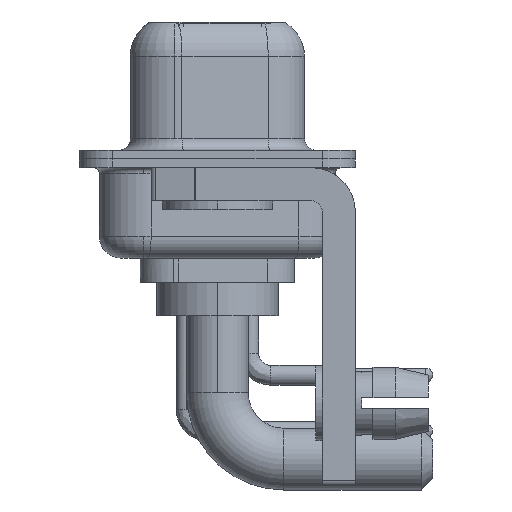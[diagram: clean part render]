
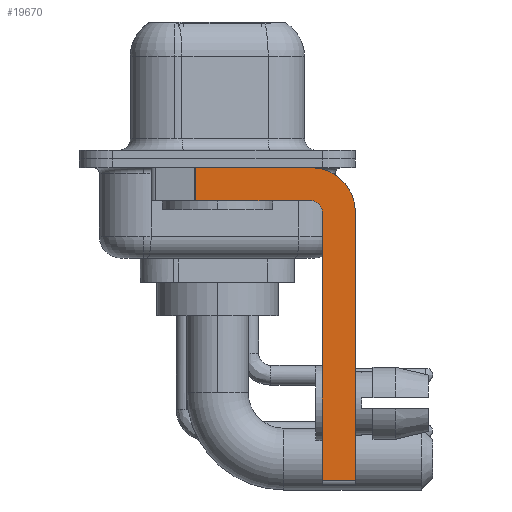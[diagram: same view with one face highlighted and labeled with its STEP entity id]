
A CAD part, left-side view. The second image highlights one B-rep face of the part: STEP entity #19670.
In plain terms, the highlighted planar face has unit normal (-1, 0, 0).
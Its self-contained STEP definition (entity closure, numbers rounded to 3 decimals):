
#291 = CARTESIAN_POINT ( 'NONE',  ( -2.9, -6.25, -14.55 ) ) ;
#1881 = DIRECTION ( 'NONE',  ( 0., 0., 1. ) ) ;
#1900 = VERTEX_POINT ( 'NONE', #3515 ) ;
#2028 = ORIENTED_EDGE ( 'NONE', *, *, #15522, .F. ) ;
#2394 = VERTEX_POINT ( 'NONE', #16954 ) ;
#2480 = VECTOR ( 'NONE', #8380, 1000. ) ;
#2775 = ORIENTED_EDGE ( 'NONE', *, *, #10385, .F. ) ;
#2887 = FACE_OUTER_BOUND ( 'NONE', #3823, .T. ) ;
#3096 = DIRECTION ( 'NONE',  ( 1., 0., 0. ) ) ;
#3515 = CARTESIAN_POINT ( 'NONE',  ( -2.9, -4.75, -2.4 ) ) ;
#3658 = ORIENTED_EDGE ( 'NONE', *, *, #13126, .T. ) ;
#3823 = EDGE_LOOP ( 'NONE', ( #15347, #6613, #8954, #4390, #16207, #3658, #2028, #2775 ) ) ;
#4247 = CARTESIAN_POINT ( 'NONE',  ( -2.9, -4.25, -0.4 ) ) ;
#4255 = VERTEX_POINT ( 'NONE', #17353 ) ;
#4303 = CARTESIAN_POINT ( 'NONE',  ( -2.9, -4.25, -2.4 ) ) ;
#4390 = ORIENTED_EDGE ( 'NONE', *, *, #6209, .F. ) ;
#4421 = DIRECTION ( 'NONE',  ( 0., 0., -1. ) ) ;
#5129 = DIRECTION ( 'NONE',  ( 0., -1., 0. ) ) ;
#5132 = VERTEX_POINT ( 'NONE', #4247 ) ;
#5274 = CARTESIAN_POINT ( 'NONE',  ( -2.9, -4.25, -1.9 ) ) ;
#5376 = VECTOR ( 'NONE', #5129, 1000. ) ;
#6014 = DIRECTION ( 'NONE',  ( 0., 0., 1. ) ) ;
#6201 = VECTOR ( 'NONE', #8021, 1000. ) ;
#6209 = EDGE_CURVE ( 'NONE', #1900, #2394, #18476, .T. ) ;
#6613 = ORIENTED_EDGE ( 'NONE', *, *, #17741, .T. ) ;
#7537 = AXIS2_PLACEMENT_3D ( 'NONE', #10836, #13992, #17464 ) ;
#7916 = VERTEX_POINT ( 'NONE', #291 ) ;
#8021 = DIRECTION ( 'NONE',  ( 0., -1., 0. ) ) ;
#8380 = DIRECTION ( 'NONE',  ( 0., 0., -1. ) ) ;
#8573 = VECTOR ( 'NONE', #1881, 1000. ) ;
#8640 = DIRECTION ( 'NONE',  ( 0., 1., 0. ) ) ;
#8706 = CARTESIAN_POINT ( 'NONE',  ( -2.9, -6.25, -2.4 ) ) ;
#8954 = ORIENTED_EDGE ( 'NONE', *, *, #16891, .F. ) ;
#9490 = AXIS2_PLACEMENT_3D ( 'NONE', #19300, #3096, #4421 ) ;
#9583 = CARTESIAN_POINT ( 'NONE',  ( -2.9, 0.978, -1.9 ) ) ;
#10385 = EDGE_CURVE ( 'NONE', #5132, #14090, #18654, .T. ) ;
#10836 = CARTESIAN_POINT ( 'NONE',  ( -2.9, -4.25, -2.4 ) ) ;
#11171 = CARTESIAN_POINT ( 'NONE',  ( -2.9, -4.25, -14.55 ) ) ;
#11282 = LINE ( 'NONE', #11171, #6201 ) ;
#11627 = EDGE_CURVE ( 'NONE', #21420, #1900, #11855, .T. ) ;
#11823 = CARTESIAN_POINT ( 'NONE',  ( -2.9, 0.978, -1.9 ) ) ;
#11855 = LINE ( 'NONE', #15225, #8573 ) ;
#13126 = EDGE_CURVE ( 'NONE', #21420, #7916, #11282, .T. ) ;
#13542 = CARTESIAN_POINT ( 'NONE',  ( -2.9, -6.25, -2.4 ) ) ;
#13663 = VECTOR ( 'NONE', #18454, 1000. ) ;
#13992 = DIRECTION ( 'NONE',  ( 1., 0., 0. ) ) ;
#14074 = LINE ( 'NONE', #5274, #16039 ) ;
#14090 = VERTEX_POINT ( 'NONE', #13542 ) ;
#14650 = AXIS2_PLACEMENT_3D ( 'NONE', #4303, #15923, #6014 ) ;
#14707 = CARTESIAN_POINT ( 'NONE',  ( -2.9, -4.75, -14.55 ) ) ;
#15225 = CARTESIAN_POINT ( 'NONE',  ( -2.9, -4.75, -14.8 ) ) ;
#15296 = LINE ( 'NONE', #11823, #13663 ) ;
#15347 = ORIENTED_EDGE ( 'NONE', *, *, #20444, .F. ) ;
#15522 = EDGE_CURVE ( 'NONE', #14090, #7916, #16763, .T. ) ;
#15923 = DIRECTION ( 'NONE',  ( -1., 0., 0. ) ) ;
#16039 = VECTOR ( 'NONE', #8640, 1000. ) ;
#16207 = ORIENTED_EDGE ( 'NONE', *, *, #11627, .F. ) ;
#16763 = LINE ( 'NONE', #8706, #2480 ) ;
#16891 = EDGE_CURVE ( 'NONE', #2394, #18814, #14074, .T. ) ;
#16954 = CARTESIAN_POINT ( 'NONE',  ( -2.9, -4.25, -1.9 ) ) ;
#17353 = CARTESIAN_POINT ( 'NONE',  ( -2.9, 0.978, -0.4 ) ) ;
#17464 = DIRECTION ( 'NONE',  ( 0., 0., -1. ) ) ;
#17741 = EDGE_CURVE ( 'NONE', #4255, #18814, #15296, .T. ) ;
#17979 = PLANE ( 'NONE',  #9490 ) ;
#18063 = CARTESIAN_POINT ( 'NONE',  ( -2.9, 3., -0.4 ) ) ;
#18454 = DIRECTION ( 'NONE',  ( 0., 0., -1. ) ) ;
#18476 = CIRCLE ( 'NONE', #14650, 0.5 ) ;
#18654 = CIRCLE ( 'NONE', #7537, 2. ) ;
#18814 = VERTEX_POINT ( 'NONE', #9583 ) ;
#19300 = CARTESIAN_POINT ( 'NONE',  ( -2.9, -4.25, -2.4 ) ) ;
#19670 = ADVANCED_FACE ( 'NONE', ( #2887 ), #17979, .F. ) ;
#20020 = LINE ( 'NONE', #18063, #5376 ) ;
#20444 = EDGE_CURVE ( 'NONE', #4255, #5132, #20020, .T. ) ;
#21420 = VERTEX_POINT ( 'NONE', #14707 ) ;
